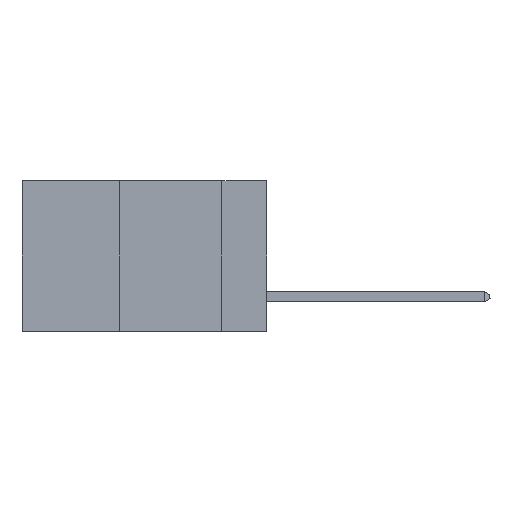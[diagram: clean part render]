
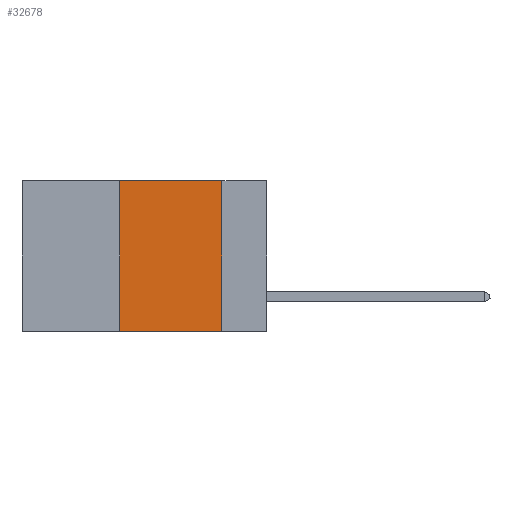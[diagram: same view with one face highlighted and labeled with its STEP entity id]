
A CAD part, left-side view. The second image highlights one B-rep face of the part: STEP entity #32678.
In plain terms, the highlighted planar face has unit normal (-1, 0, 0).
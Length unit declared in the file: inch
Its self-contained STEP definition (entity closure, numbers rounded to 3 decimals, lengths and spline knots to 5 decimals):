
#1917 = CARTESIAN_POINT ( 'NONE',  ( 0., 0.6, 0. ) ) ;
#2166 = VERTEX_POINT ( 'NONE', #11044 ) ;
#3049 = CARTESIAN_POINT ( 'NONE',  ( 0., 0.6, -0.37 ) ) ;
#4167 = CARTESIAN_POINT ( 'NONE',  ( 0., 0.11, 0. ) ) ;
#5173 = CARTESIAN_POINT ( 'NONE',  ( 0., 0.36, 0. ) ) ;
#5548 = VERTEX_POINT ( 'NONE', #17329 ) ;
#7317 = LINE ( 'NONE', #1917, #13499 ) ;
#8099 = DIRECTION ( 'NONE',  ( 0., 0., 1. ) ) ;
#8263 = VECTOR ( 'NONE', #8099, 39.37008 ) ;
#9656 = LINE ( 'NONE', #4167, #19393 ) ;
#9923 = FACE_OUTER_BOUND ( 'NONE', #21233, .T. ) ;
#10056 = EDGE_CURVE ( 'NONE', #2166, #25071, #9656, .T. ) ;
#11044 = CARTESIAN_POINT ( 'NONE',  ( 0., 0.11, 0. ) ) ;
#13100 = LINE ( 'NONE', #5173, #8263 ) ;
#13372 = VECTOR ( 'NONE', #28066, 39.37008 ) ;
#13499 = VECTOR ( 'NONE', #32780, 39.37008 ) ;
#14135 = ORIENTED_EDGE ( 'NONE', *, *, #23092, .F. ) ;
#15287 = PLANE ( 'NONE',  #32387 ) ;
#16181 = CARTESIAN_POINT ( 'NONE',  ( 0., 0.6, 0. ) ) ;
#16353 = ORIENTED_EDGE ( 'NONE', *, *, #23684, .F. ) ;
#16780 = CARTESIAN_POINT ( 'NONE',  ( 0., 0.36, -0.37 ) ) ;
#17329 = CARTESIAN_POINT ( 'NONE',  ( 0., 0.36, 0. ) ) ;
#18107 = DIRECTION ( 'NONE',  ( 0., 0., -1. ) ) ;
#19393 = VECTOR ( 'NONE', #18107, 39.37008 ) ;
#19855 = CARTESIAN_POINT ( 'NONE',  ( 0., 0.11, -0.37 ) ) ;
#21233 = EDGE_LOOP ( 'NONE', ( #31883, #16353, #14135, #26443 ) ) ;
#22103 = VERTEX_POINT ( 'NONE', #16780 ) ;
#23092 = EDGE_CURVE ( 'NONE', #22103, #5548, #13100, .T. ) ;
#23684 = EDGE_CURVE ( 'NONE', #5548, #2166, #7317, .T. ) ;
#25071 = VERTEX_POINT ( 'NONE', #19855 ) ;
#25220 = DIRECTION ( 'NONE',  ( 1., 0., 0. ) ) ;
#26443 = ORIENTED_EDGE ( 'NONE', *, *, #34322, .T. ) ;
#28066 = DIRECTION ( 'NONE',  ( 0., -1., 0. ) ) ;
#28157 = DIRECTION ( 'NONE',  ( 0., 0., -1. ) ) ;
#28391 = LINE ( 'NONE', #3049, #13372 ) ;
#31883 = ORIENTED_EDGE ( 'NONE', *, *, #10056, .F. ) ;
#32387 = AXIS2_PLACEMENT_3D ( 'NONE', #16181, #25220, #28157 ) ;
#32678 = ADVANCED_FACE ( 'NONE', ( #9923 ), #15287, .F. ) ;
#32780 = DIRECTION ( 'NONE',  ( 0., -1., 0. ) ) ;
#34322 = EDGE_CURVE ( 'NONE', #22103, #25071, #28391, .T. ) ;
